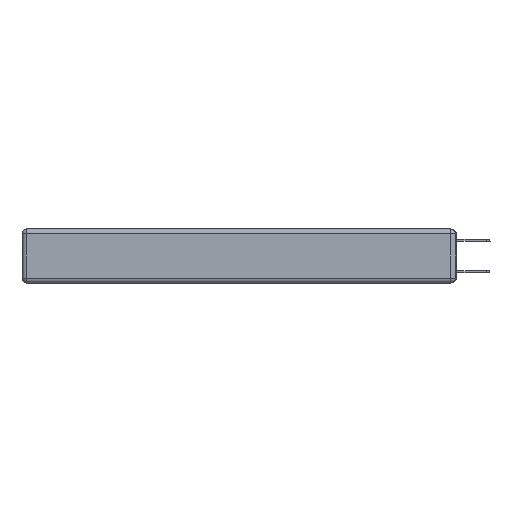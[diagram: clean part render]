
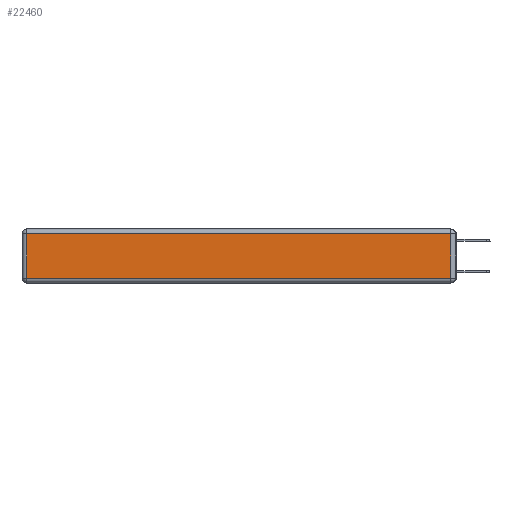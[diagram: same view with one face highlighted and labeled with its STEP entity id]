
A CAD part, left-side view. The second image highlights one B-rep face of the part: STEP entity #22460.
In plain terms, the highlighted planar face has unit normal (-1, 0, 0).
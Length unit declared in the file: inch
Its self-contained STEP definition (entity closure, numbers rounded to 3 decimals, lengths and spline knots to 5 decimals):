
#366 = DIRECTION ( 'NONE',  ( -1., 0., 0. ) ) ;
#924 = CARTESIAN_POINT ( 'NONE',  ( 0., 0.03, -0.03 ) ) ;
#1152 = DIRECTION ( 'NONE',  ( 0., 1., 0. ) ) ;
#1439 = ORIENTED_EDGE ( 'NONE', *, *, #10945, .T. ) ;
#2428 = ORIENTED_EDGE ( 'NONE', *, *, #17513, .T. ) ;
#3711 = LINE ( 'NONE', #4605, #16762 ) ;
#4309 = VERTEX_POINT ( 'NONE', #8017 ) ;
#4605 = CARTESIAN_POINT ( 'NONE',  ( 0., 0.03, -0.343 ) ) ;
#4661 = DIRECTION ( 'NONE',  ( 0., 0., 1. ) ) ;
#4790 = DIRECTION ( 'NONE',  ( 0., 0., -1. ) ) ;
#6659 = DIRECTION ( 'NONE',  ( 0., -1., 0. ) ) ;
#7348 = CARTESIAN_POINT ( 'NONE',  ( 0., 2.72, -0.03 ) ) ;
#8017 = CARTESIAN_POINT ( 'NONE',  ( 0., 0.03, -0.313 ) ) ;
#8513 = VECTOR ( 'NONE', #1152, 39.37008 ) ;
#8774 = VECTOR ( 'NONE', #4790, 39.37008 ) ;
#8850 = EDGE_CURVE ( 'NONE', #24586, #17068, #17702, .T. ) ;
#8864 = CARTESIAN_POINT ( 'NONE',  ( 0., 2.72, -0.343 ) ) ;
#9549 = EDGE_LOOP ( 'NONE', ( #22590, #1439, #2428, #19524 ) ) ;
#10945 = EDGE_CURVE ( 'NONE', #4309, #20372, #3711, .T. ) ;
#11384 = CARTESIAN_POINT ( 'NONE',  ( 0., 2.75, -0.03 ) ) ;
#13367 = EDGE_CURVE ( 'NONE', #17068, #4309, #25199, .T. ) ;
#14857 = CARTESIAN_POINT ( 'NONE',  ( 0., 0., -0.313 ) ) ;
#15553 = LINE ( 'NONE', #11384, #8513 ) ;
#16762 = VECTOR ( 'NONE', #17061, 39.37008 ) ;
#17061 = DIRECTION ( 'NONE',  ( 0., 0., 1. ) ) ;
#17068 = VERTEX_POINT ( 'NONE', #18371 ) ;
#17513 = EDGE_CURVE ( 'NONE', #20372, #24586, #15553, .T. ) ;
#17702 = LINE ( 'NONE', #8864, #8774 ) ;
#18371 = CARTESIAN_POINT ( 'NONE',  ( 0., 2.72, -0.313 ) ) ;
#18447 = AXIS2_PLACEMENT_3D ( 'NONE', #20606, #366, #4661 ) ;
#19524 = ORIENTED_EDGE ( 'NONE', *, *, #8850, .T. ) ;
#19583 = FACE_OUTER_BOUND ( 'NONE', #9549, .T. ) ;
#20372 = VERTEX_POINT ( 'NONE', #924 ) ;
#20606 = CARTESIAN_POINT ( 'NONE',  ( 0., 0., -0.343 ) ) ;
#21392 = VECTOR ( 'NONE', #6659, 39.37008 ) ;
#22460 = ADVANCED_FACE ( 'NONE', ( #19583 ), #22813, .T. ) ;
#22590 = ORIENTED_EDGE ( 'NONE', *, *, #13367, .T. ) ;
#22813 = PLANE ( 'NONE',  #18447 ) ;
#24586 = VERTEX_POINT ( 'NONE', #7348 ) ;
#25199 = LINE ( 'NONE', #14857, #21392 ) ;
